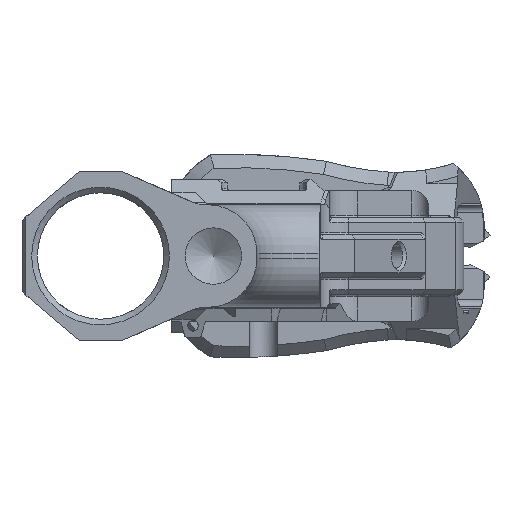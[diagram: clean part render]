
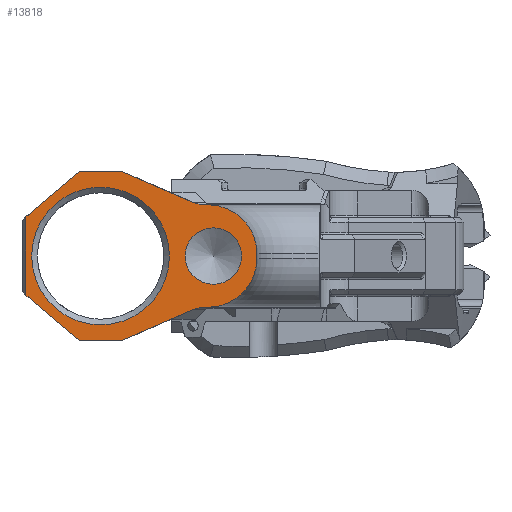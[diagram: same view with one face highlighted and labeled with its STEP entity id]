
A CAD part, left-side view. The second image highlights one B-rep face of the part: STEP entity #13818.
In plain terms, the highlighted planar face has unit normal (-1, 0, 0).
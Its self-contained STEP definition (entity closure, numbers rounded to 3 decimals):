
#156=FACE_BOUND('',#4442,.T.);
#157=FACE_BOUND('',#4443,.T.);
#1119=LINE('',#23762,#2302);
#1186=LINE('',#25580,#2369);
#1187=LINE('',#25582,#2370);
#1188=LINE('',#25584,#2371);
#1189=LINE('',#25586,#2372);
#1190=LINE('',#25588,#2373);
#1191=LINE('',#25590,#2374);
#1192=LINE('',#25592,#2375);
#1193=LINE('',#25594,#2376);
#1194=LINE('',#25596,#2377);
#1195=LINE('',#25603,#2378);
#1196=LINE('',#25608,#2379);
#2302=VECTOR('',#17011,1000.);
#2369=VECTOR('',#17212,1000.);
#2370=VECTOR('',#17213,1000.);
#2371=VECTOR('',#17214,1000.);
#2372=VECTOR('',#17215,1000.);
#2373=VECTOR('',#17216,1000.);
#2374=VECTOR('',#17217,1000.);
#2375=VECTOR('',#17218,1000.);
#2376=VECTOR('',#17219,1000.);
#2377=VECTOR('',#17220,1000.);
#2378=VECTOR('',#17227,1000.);
#2379=VECTOR('',#17232,1000.);
#3126=PLANE('',#14858);
#3646=FACE_OUTER_BOUND('',#4441,.T.);
#4441=EDGE_LOOP('',(#11150,#11151,#11152,#11153,#11154,#11155,#11156,#11157,
#11158,#11159,#11160,#11161,#11162,#11163,#11164,#11165,#11166,#11167));
#4442=EDGE_LOOP('',(#11168));
#4443=EDGE_LOOP('',(#11169));
#5510=CIRCLE('',#14859,7.112);
#5511=CIRCLE('',#14860,7.112);
#5512=CIRCLE('',#14861,3.175);
#5513=CIRCLE('',#14862,10.922);
#5514=CIRCLE('',#14863,10.922);
#5515=CIRCLE('',#14864,3.175);
#5516=CIRCLE('',#14865,6.35);
#5517=CIRCLE('',#14866,15.494);
#6429=VERTEX_POINT('',#23759);
#6430=VERTEX_POINT('',#23761);
#6557=VERTEX_POINT('',#25576);
#6558=VERTEX_POINT('',#25577);
#6559=VERTEX_POINT('',#25579);
#6560=VERTEX_POINT('',#25581);
#6561=VERTEX_POINT('',#25583);
#6562=VERTEX_POINT('',#25585);
#6563=VERTEX_POINT('',#25587);
#6564=VERTEX_POINT('',#25589);
#6565=VERTEX_POINT('',#25591);
#6566=VERTEX_POINT('',#25593);
#6567=VERTEX_POINT('',#25595);
#6568=VERTEX_POINT('',#25598);
#6569=VERTEX_POINT('',#25600);
#6570=VERTEX_POINT('',#25602);
#6571=VERTEX_POINT('',#25604);
#6572=VERTEX_POINT('',#25606);
#6573=VERTEX_POINT('',#25609);
#6574=VERTEX_POINT('',#25611);
#8081=EDGE_CURVE('',#6430,#6429,#1119,.T.);
#8237=EDGE_CURVE('',#6557,#6558,#5510,.T.);
#8238=EDGE_CURVE('',#6558,#6559,#1186,.T.);
#8239=EDGE_CURVE('',#6559,#6560,#1187,.T.);
#8240=EDGE_CURVE('',#6560,#6561,#1188,.T.);
#8241=EDGE_CURVE('',#6562,#6561,#1189,.T.);
#8242=EDGE_CURVE('',#6562,#6563,#1190,.T.);
#8243=EDGE_CURVE('',#6564,#6563,#1191,.T.);
#8244=EDGE_CURVE('',#6564,#6565,#1192,.T.);
#8245=EDGE_CURVE('',#6565,#6566,#1193,.T.);
#8246=EDGE_CURVE('',#6567,#6566,#1194,.T.);
#8247=EDGE_CURVE('',#6567,#6430,#5511,.T.);
#8248=EDGE_CURVE('',#6429,#6568,#5512,.F.);
#8249=EDGE_CURVE('',#6568,#6569,#5513,.T.);
#8250=EDGE_CURVE('',#6570,#6569,#1195,.T.);
#8251=EDGE_CURVE('',#6570,#6571,#5514,.T.);
#8252=EDGE_CURVE('',#6571,#6572,#5515,.F.);
#8253=EDGE_CURVE('',#6572,#6557,#1196,.T.);
#8254=EDGE_CURVE('',#6573,#6573,#5516,.T.);
#8255=EDGE_CURVE('',#6574,#6574,#5517,.T.);
#11150=ORIENTED_EDGE('',*,*,#8237,.T.);
#11151=ORIENTED_EDGE('',*,*,#8238,.T.);
#11152=ORIENTED_EDGE('',*,*,#8239,.T.);
#11153=ORIENTED_EDGE('',*,*,#8240,.T.);
#11154=ORIENTED_EDGE('',*,*,#8241,.F.);
#11155=ORIENTED_EDGE('',*,*,#8242,.T.);
#11156=ORIENTED_EDGE('',*,*,#8243,.F.);
#11157=ORIENTED_EDGE('',*,*,#8244,.T.);
#11158=ORIENTED_EDGE('',*,*,#8245,.T.);
#11159=ORIENTED_EDGE('',*,*,#8246,.F.);
#11160=ORIENTED_EDGE('',*,*,#8247,.T.);
#11161=ORIENTED_EDGE('',*,*,#8081,.T.);
#11162=ORIENTED_EDGE('',*,*,#8248,.T.);
#11163=ORIENTED_EDGE('',*,*,#8249,.T.);
#11164=ORIENTED_EDGE('',*,*,#8250,.F.);
#11165=ORIENTED_EDGE('',*,*,#8251,.T.);
#11166=ORIENTED_EDGE('',*,*,#8252,.T.);
#11167=ORIENTED_EDGE('',*,*,#8253,.T.);
#11168=ORIENTED_EDGE('',*,*,#8254,.F.);
#11169=ORIENTED_EDGE('',*,*,#8255,.T.);
#13818=ADVANCED_FACE('',(#3646,#156,#157),#3126,.T.);
#14858=AXIS2_PLACEMENT_3D('',#25575,#17208,#17209);
#14859=AXIS2_PLACEMENT_3D('',#25578,#17210,#17211);
#14860=AXIS2_PLACEMENT_3D('',#25597,#17221,#17222);
#14861=AXIS2_PLACEMENT_3D('',#25599,#17223,#17224);
#14862=AXIS2_PLACEMENT_3D('',#25601,#17225,#17226);
#14863=AXIS2_PLACEMENT_3D('',#25605,#17228,#17229);
#14864=AXIS2_PLACEMENT_3D('',#25607,#17230,#17231);
#14865=AXIS2_PLACEMENT_3D('',#25610,#17233,#17234);
#14866=AXIS2_PLACEMENT_3D('',#25612,#17235,#17236);
#17011=DIRECTION('',(0.,-1.,0.));
#17208=DIRECTION('center_axis',(-1.,0.,0.));
#17209=DIRECTION('ref_axis',(0.,1.,0.));
#17210=DIRECTION('center_axis',(1.,0.,0.));
#17211=DIRECTION('ref_axis',(0.,0.,
1.));
#17212=DIRECTION('',(0.,0.917,0.399));
#17213=DIRECTION('',(0.,1.,0.));
#17214=DIRECTION('',(0.,0.762,-0.647));
#17215=DIRECTION('',(0.,-0.759,0.652));
#17216=DIRECTION('',(0.,0.,-1.));
#17217=DIRECTION('',(0.,0.759,0.652));
#17218=DIRECTION('',(0.,-0.762,-0.647));
#17219=DIRECTION('',(0.,-1.,0.));
#17220=DIRECTION('',(0.,0.917,-0.399));
#17221=DIRECTION('center_axis',(1.,0.,0.));
#17222=DIRECTION('ref_axis',(0.,0.,
-1.));
#17223=DIRECTION('center_axis',(-1.,0.,0.));
#17224=DIRECTION('ref_axis',(0.,0.,1.));
#17225=DIRECTION('center_axis',(-1.,0.,0.));
#17226=DIRECTION('ref_axis',(0.,0.,
-1.));
#17227=DIRECTION('',(0.,0.,-1.));
#17228=DIRECTION('center_axis',(-1.,0.,0.));
#17229=DIRECTION('ref_axis',(0.,-1.,0.));
#17230=DIRECTION('center_axis',(-1.,0.,0.));
#17231=DIRECTION('ref_axis',(0.,0.,1.));
#17232=DIRECTION('',(0.,1.,0.));
#17233=DIRECTION('center_axis',(-1.,0.,0.));
#17234=DIRECTION('ref_axis',(0.,1.,0.));
#17235=DIRECTION('center_axis',(1.,0.,0.));
#17236=DIRECTION('ref_axis',(0.,0.,
1.));
#23759=CARTESIAN_POINT('',(-190.86,49.409,-53.584));
#23761=CARTESIAN_POINT('',(-190.86,50.38,-53.584));
#23762=CARTESIAN_POINT('',(-190.86,-21.671,-53.584));
#25575=CARTESIAN_POINT('Origin',(-190.86,-10.077,-30.571));
#25576=CARTESIAN_POINT('',(-190.86,50.38,-30.571));
#25577=CARTESIAN_POINT('',(-190.86,53.216,-29.981));
#25578=CARTESIAN_POINT('Origin',(-190.86,50.38,-23.459));
#25579=CARTESIAN_POINT('',(-190.86,69.209,-23.027));
#25580=CARTESIAN_POINT('',(-190.86,69.015,-23.112));
#25581=CARTESIAN_POINT('',(-190.86,78.734,-23.027));
#25582=CARTESIAN_POINT('',(-190.86,69.209,-23.027));
#25583=CARTESIAN_POINT('',(-190.86,87.51,-30.474));
#25584=CARTESIAN_POINT('',(-190.86,78.734,-23.027));
#25585=CARTESIAN_POINT('',(-190.86,90.761,-33.267));
#25586=CARTESIAN_POINT('',(-190.86,90.761,-33.267));
#25587=CARTESIAN_POINT('',(-190.86,90.761,-50.888));
#25588=CARTESIAN_POINT('',(-190.86,90.761,-33.267));
#25589=CARTESIAN_POINT('',(-190.86,87.51,-53.681));
#25590=CARTESIAN_POINT('',(-190.86,87.51,-53.681));
#25591=CARTESIAN_POINT('',(-190.86,78.734,-61.127));
#25592=CARTESIAN_POINT('',(-190.86,87.51,-53.681));
#25593=CARTESIAN_POINT('',(-190.86,69.209,-61.127));
#25594=CARTESIAN_POINT('',(-190.86,78.734,-61.127));
#25595=CARTESIAN_POINT('',(-190.86,53.216,-54.173));
#25596=CARTESIAN_POINT('',(-190.86,69.015,-61.043));
#25597=CARTESIAN_POINT('Origin',(-190.86,50.38,-60.696));
#25598=CARTESIAN_POINT('',(-190.86,49.252,-53.573));
#25599=CARTESIAN_POINT('Origin',(-190.86,49.11,-56.744));
#25600=CARTESIAN_POINT('',(-190.86,38.818,-42.662));
#25601=CARTESIAN_POINT('Origin',(-190.86,49.74,-42.662));
#25602=CARTESIAN_POINT('',(-190.86,38.818,-41.493));
#25603=CARTESIAN_POINT('',(-190.86,38.818,-41.493));
#25604=CARTESIAN_POINT('',(-190.86,49.252,-30.582));
#25605=CARTESIAN_POINT('Origin',(-190.86,49.74,-41.493));
#25606=CARTESIAN_POINT('',(-190.86,49.409,-30.571));
#25607=CARTESIAN_POINT('Origin',(-190.86,49.11,-27.41));
#25608=CARTESIAN_POINT('',(-190.86,50.38,-30.571));
#25609=CARTESIAN_POINT('',(-190.86,54.947,-42.077));
#25610=CARTESIAN_POINT('Origin',(-190.86,48.597,-42.077));
#25611=CARTESIAN_POINT('',(-190.86,73.972,-57.571));
#25612=CARTESIAN_POINT('Origin',(-190.86,73.972,-42.077));
